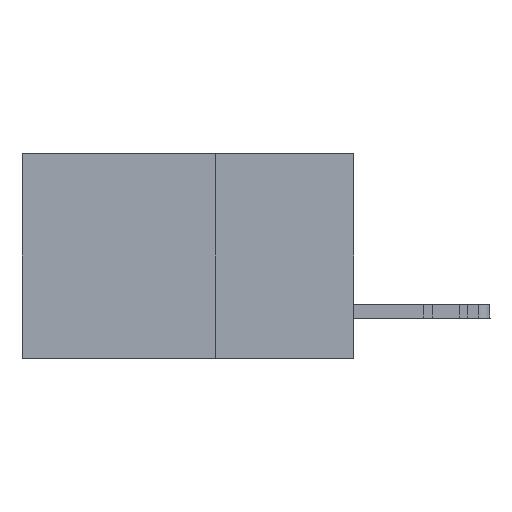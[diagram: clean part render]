
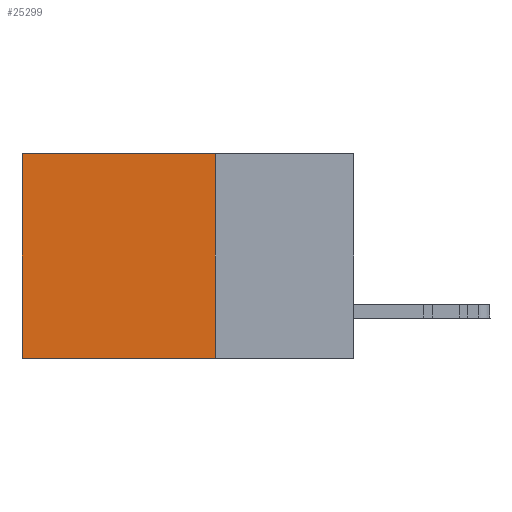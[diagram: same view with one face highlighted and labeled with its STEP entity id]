
A CAD part, left-side view. The second image highlights one B-rep face of the part: STEP entity #25299.
In plain terms, the highlighted planar face has unit normal (-1, 0, 0).
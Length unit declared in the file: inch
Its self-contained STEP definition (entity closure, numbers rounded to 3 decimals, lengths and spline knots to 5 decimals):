
#6 = CARTESIAN_POINT ( 'NONE',  ( 0.2875, 0.25, 0. ) ) ;
#760 = DIRECTION ( 'NONE',  ( 1., 0., 0. ) ) ;
#2400 = LINE ( 'NONE', #26791, #9971 ) ;
#2807 = EDGE_CURVE ( 'NONE', #13890, #38024, #24010, .T. ) ;
#5147 = FACE_OUTER_BOUND ( 'NONE', #9985, .T. ) ;
#5718 = ORIENTED_EDGE ( 'NONE', *, *, #2807, .F. ) ;
#8723 = CARTESIAN_POINT ( 'NONE',  ( 0.2875, 0.25, 0. ) ) ;
#9971 = VECTOR ( 'NONE', #17065, 39.37008 ) ;
#9985 = EDGE_LOOP ( 'NONE', ( #31405, #20683, #5718, #22049 ) ) ;
#10071 = AXIS2_PLACEMENT_3D ( 'NONE', #10340, #760, #23266 ) ;
#10151 = LINE ( 'NONE', #16162, #26219 ) ;
#10340 = CARTESIAN_POINT ( 'NONE',  ( 0.2875, 0.25, 0. ) ) ;
#11397 = VERTEX_POINT ( 'NONE', #39331 ) ;
#11525 = VERTEX_POINT ( 'NONE', #33569 ) ;
#13537 = PLANE ( 'NONE',  #10071 ) ;
#13890 = VERTEX_POINT ( 'NONE', #8723 ) ;
#14822 = LINE ( 'NONE', #6, #39238 ) ;
#15395 = VECTOR ( 'NONE', #23394, 39.37008 ) ;
#16162 = CARTESIAN_POINT ( 'NONE',  ( 0.2875, 0.25, -0.37 ) ) ;
#17065 = DIRECTION ( 'NONE',  ( 0., 0., -1. ) ) ;
#19096 = EDGE_CURVE ( 'NONE', #38024, #11397, #10151, .T. ) ;
#20107 = CARTESIAN_POINT ( 'NONE',  ( 0.2875, 0.25, 0. ) ) ;
#20683 = ORIENTED_EDGE ( 'NONE', *, *, #19096, .F. ) ;
#20905 = CARTESIAN_POINT ( 'NONE',  ( 0.2875, 0.25, -0.37 ) ) ;
#22049 = ORIENTED_EDGE ( 'NONE', *, *, #23962, .T. ) ;
#23266 = DIRECTION ( 'NONE',  ( 0., 0., -1. ) ) ;
#23394 = DIRECTION ( 'NONE',  ( 0., 0., -1. ) ) ;
#23962 = EDGE_CURVE ( 'NONE', #13890, #11525, #14822, .T. ) ;
#24010 = LINE ( 'NONE', #20107, #15395 ) ;
#25299 = ADVANCED_FACE ( 'NONE', ( #5147 ), #13537, .F. ) ;
#26219 = VECTOR ( 'NONE', #28969, 39.37008 ) ;
#26791 = CARTESIAN_POINT ( 'NONE',  ( 0.2875, 0.6, 0. ) ) ;
#28969 = DIRECTION ( 'NONE',  ( 0., 1., 0. ) ) ;
#31405 = ORIENTED_EDGE ( 'NONE', *, *, #32431, .T. ) ;
#32431 = EDGE_CURVE ( 'NONE', #11525, #11397, #2400, .T. ) ;
#33569 = CARTESIAN_POINT ( 'NONE',  ( 0.2875, 0.6, 0. ) ) ;
#35178 = DIRECTION ( 'NONE',  ( 0., 1., 0. ) ) ;
#38024 = VERTEX_POINT ( 'NONE', #20905 ) ;
#39238 = VECTOR ( 'NONE', #35178, 39.37008 ) ;
#39331 = CARTESIAN_POINT ( 'NONE',  ( 0.2875, 0.6, -0.37 ) ) ;
